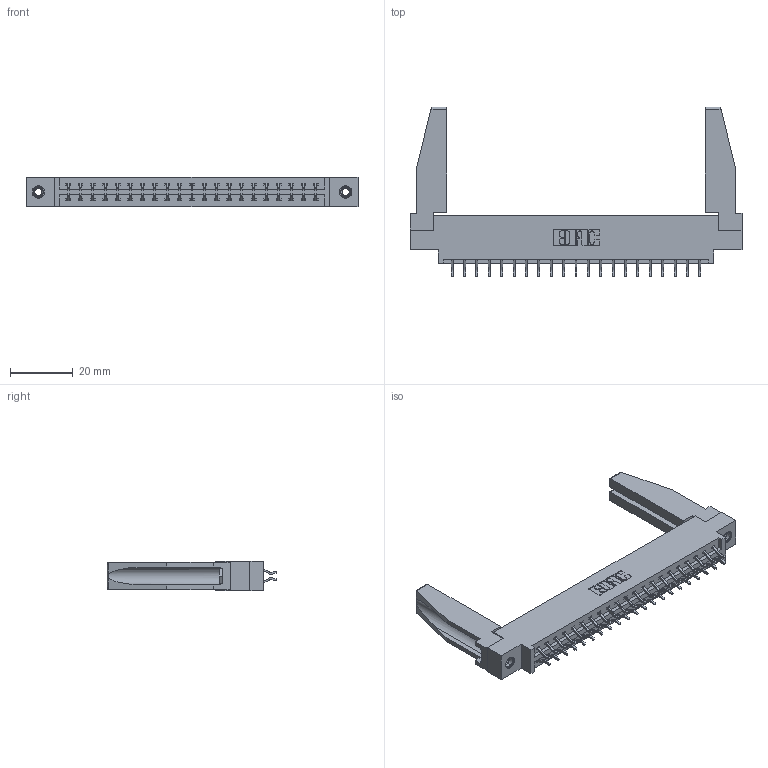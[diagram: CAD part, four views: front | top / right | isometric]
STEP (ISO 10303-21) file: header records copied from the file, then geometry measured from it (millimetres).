
FILE_DESCRIPTION (( 'STEP AP203' ), '1' );
FILE_NAME ('387-042-556-878.STEP', '2019-10-18T04:41:47', ( '' ), ( '' ), 'SwSTEP 2.0', 'SolidWorks 2016', '' );
FILE_SCHEMA (( 'CONFIG_CONTROL_DESIGN' ));
Length unit declared in the file: inch
Products named in the file (5): 337 Part_0.170 Offset - 0.156 Dia-TI; 345-292-001_556 Tail; 345-250-001_345-250-001-102; 387-042-556-878; 307-220-078
Assembly tree (47 placements, depth 2):
  387-042-556-878
    337 Part_0.170 Offset - 0.156 Dia-TI
    345-292-001_556 Tail  x42
    345-250-001_345-250-001-102  x2
    307-220-078  x2
Bounding box: 106.22 x 54.37 x 9.4 mm (x, y, z)
Volume: 14789.2 mm3; surface area: 15894.8 mm2
Topology: 47 solids, 47 shells, 2768 faces, 8171 edges, 5382 vertices
Faces by surface type: plane 1922, cylinder 830, cone 12, torus 4
Entity records: 21790 total; most frequent: CARTESIAN_POINT 3704, ORIENTED_EDGE 3584, DIRECTION 3184, EDGE_CURVE 1792, LINE 1618, VECTOR 1618, VERTEX_POINT 1188, AXIS2_PLACEMENT_3D 783
